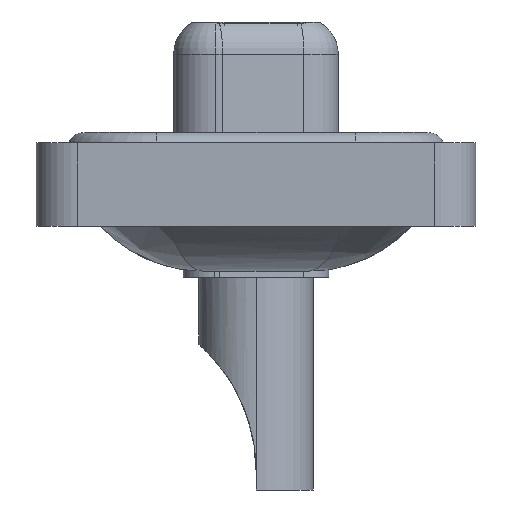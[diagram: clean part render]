
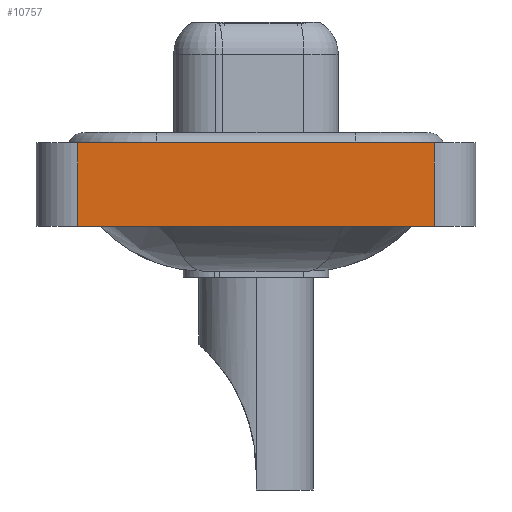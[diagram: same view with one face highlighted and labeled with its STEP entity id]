
A CAD part, left-side view. The second image highlights one B-rep face of the part: STEP entity #10757.
In plain terms, the highlighted planar face has unit normal (-1, 0, 0).
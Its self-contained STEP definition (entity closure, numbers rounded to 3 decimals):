
#112 = CARTESIAN_POINT ( 'NONE',  ( -7.25, -8.55, -3.6 ) ) ;
#503 = ORIENTED_EDGE ( 'NONE', *, *, #14486, .F. ) ;
#1427 = FACE_OUTER_BOUND ( 'NONE', #13301, .T. ) ;
#2631 = VERTEX_POINT ( 'NONE', #9219 ) ;
#4036 = DIRECTION ( 'NONE',  ( 0., 0., 1. ) ) ;
#4145 = LINE ( 'NONE', #5527, #7898 ) ;
#4745 = ORIENTED_EDGE ( 'NONE', *, *, #5090, .T. ) ;
#4787 = CARTESIAN_POINT ( 'NONE',  ( -7.25, -8.55, -3.6 ) ) ;
#5090 = EDGE_CURVE ( 'NONE', #13004, #11810, #4145, .T. ) ;
#5202 = CARTESIAN_POINT ( 'NONE',  ( -7.25, 8.55, 0.4 ) ) ;
#5527 = CARTESIAN_POINT ( 'NONE',  ( -7.25, -8.55, -3.6 ) ) ;
#5737 = CARTESIAN_POINT ( 'NONE',  ( -7.25, -8.55, 0.4 ) ) ;
#5783 = CARTESIAN_POINT ( 'NONE',  ( -7.25, -8.55, 0.4 ) ) ;
#7898 = VECTOR ( 'NONE', #9623, 1000. ) ;
#7931 = PLANE ( 'NONE',  #13387 ) ;
#8071 = LINE ( 'NONE', #5737, #8372 ) ;
#8168 = DIRECTION ( 'NONE',  ( 0., -1., 0. ) ) ;
#8372 = VECTOR ( 'NONE', #16399, 1000. ) ;
#8913 = EDGE_CURVE ( 'NONE', #2631, #13004, #10999, .T. ) ;
#9219 = CARTESIAN_POINT ( 'NONE',  ( -7.25, 8.55, -3.6 ) ) ;
#9576 = CARTESIAN_POINT ( 'NONE',  ( -7.25, -8.55, -3.6 ) ) ;
#9623 = DIRECTION ( 'NONE',  ( 0., 0., 1. ) ) ;
#9626 = VECTOR ( 'NONE', #8168, 1000. ) ;
#10757 = ADVANCED_FACE ( 'NONE', ( #1427 ), #7931, .T. ) ;
#10927 = DIRECTION ( 'NONE',  ( -1., 0., 0. ) ) ;
#10999 = LINE ( 'NONE', #9576, #9626 ) ;
#11810 = VERTEX_POINT ( 'NONE', #5783 ) ;
#12497 = CARTESIAN_POINT ( 'NONE',  ( -7.25, 8.55, -3.6 ) ) ;
#13004 = VERTEX_POINT ( 'NONE', #4787 ) ;
#13211 = VERTEX_POINT ( 'NONE', #5202 ) ;
#13301 = EDGE_LOOP ( 'NONE', ( #4745, #13433, #503, #14316 ) ) ;
#13387 = AXIS2_PLACEMENT_3D ( 'NONE', #112, #10927, #4036 ) ;
#13433 = ORIENTED_EDGE ( 'NONE', *, *, #13773, .F. ) ;
#13773 = EDGE_CURVE ( 'NONE', #13211, #11810, #8071, .T. ) ;
#14316 = ORIENTED_EDGE ( 'NONE', *, *, #8913, .T. ) ;
#14486 = EDGE_CURVE ( 'NONE', #2631, #13211, #16357, .T. ) ;
#15849 = VECTOR ( 'NONE', #16611, 1000. ) ;
#16357 = LINE ( 'NONE', #12497, #15849 ) ;
#16399 = DIRECTION ( 'NONE',  ( 0., -1., 0. ) ) ;
#16611 = DIRECTION ( 'NONE',  ( 0., 0., 1. ) ) ;
